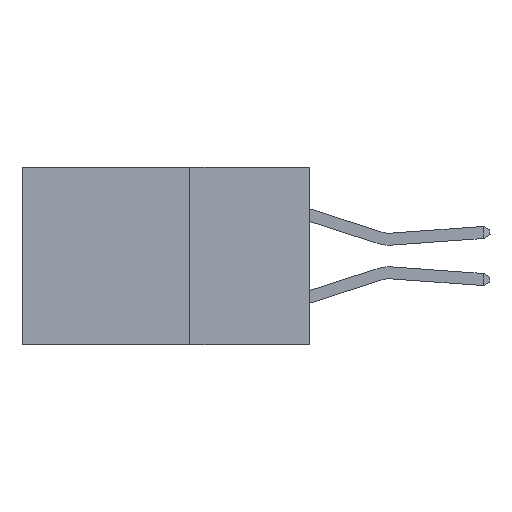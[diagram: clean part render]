
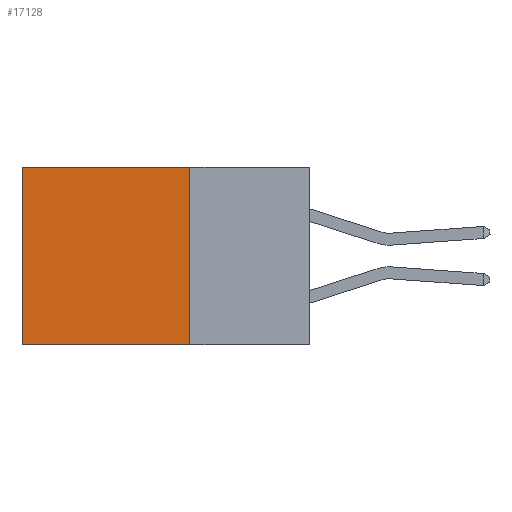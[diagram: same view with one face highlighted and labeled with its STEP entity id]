
A CAD part, left-side view. The second image highlights one B-rep face of the part: STEP entity #17128.
In plain terms, the highlighted planar face has unit normal (-1, 0, 0).
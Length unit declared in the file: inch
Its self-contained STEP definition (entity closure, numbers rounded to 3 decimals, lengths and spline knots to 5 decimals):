
#184 = LINE ( 'NONE', #22517, #8501 ) ;
#696 = CARTESIAN_POINT ( 'NONE',  ( 0.298, 0.6, 0. ) ) ;
#2286 = EDGE_CURVE ( 'NONE', #18534, #9116, #24153, .T. ) ;
#2993 = DIRECTION ( 'NONE',  ( 0., 0., -1. ) ) ;
#3890 = DIRECTION ( 'NONE',  ( 0., 0., -1. ) ) ;
#3920 = VECTOR ( 'NONE', #28299, 39.37008 ) ;
#4253 = EDGE_LOOP ( 'NONE', ( #7349, #31190, #12575, #24698 ) ) ;
#7349 = ORIENTED_EDGE ( 'NONE', *, *, #2286, .T. ) ;
#8501 = VECTOR ( 'NONE', #25023, 39.37008 ) ;
#9116 = VERTEX_POINT ( 'NONE', #18251 ) ;
#9934 = EDGE_CURVE ( 'NONE', #31045, #18534, #184, .T. ) ;
#10571 = CARTESIAN_POINT ( 'NONE',  ( 0.298, 0.25, 0. ) ) ;
#11083 = AXIS2_PLACEMENT_3D ( 'NONE', #10571, #18210, #2993 ) ;
#12575 = ORIENTED_EDGE ( 'NONE', *, *, #26874, .F. ) ;
#14338 = FACE_OUTER_BOUND ( 'NONE', #4253, .T. ) ;
#14443 = CARTESIAN_POINT ( 'NONE',  ( 0.298, 0.25, -0.37 ) ) ;
#15634 = PLANE ( 'NONE',  #11083 ) ;
#17128 = ADVANCED_FACE ( 'NONE', ( #14338 ), #15634, .F. ) ;
#17450 = VECTOR ( 'NONE', #3890, 39.37008 ) ;
#18210 = DIRECTION ( 'NONE',  ( 1., 0., 0. ) ) ;
#18235 = CARTESIAN_POINT ( 'NONE',  ( 0.298, 0.6, 0. ) ) ;
#18249 = LINE ( 'NONE', #19089, #17450 ) ;
#18251 = CARTESIAN_POINT ( 'NONE',  ( 0.298, 0.6, -0.37 ) ) ;
#18534 = VERTEX_POINT ( 'NONE', #18235 ) ;
#19089 = CARTESIAN_POINT ( 'NONE',  ( 0.298, 0.25, 0. ) ) ;
#21722 = VECTOR ( 'NONE', #27065, 39.37008 ) ;
#22517 = CARTESIAN_POINT ( 'NONE',  ( 0.298, 0.25, 0. ) ) ;
#22523 = LINE ( 'NONE', #14443, #21722 ) ;
#24153 = LINE ( 'NONE', #696, #3920 ) ;
#24698 = ORIENTED_EDGE ( 'NONE', *, *, #9934, .T. ) ;
#25023 = DIRECTION ( 'NONE',  ( 0., 1., 0. ) ) ;
#26874 = EDGE_CURVE ( 'NONE', #31045, #28324, #18249, .T. ) ;
#27065 = DIRECTION ( 'NONE',  ( 0., 1., 0. ) ) ;
#28202 = EDGE_CURVE ( 'NONE', #28324, #9116, #22523, .T. ) ;
#28299 = DIRECTION ( 'NONE',  ( 0., 0., -1. ) ) ;
#28324 = VERTEX_POINT ( 'NONE', #30113 ) ;
#29826 = CARTESIAN_POINT ( 'NONE',  ( 0.298, 0.25, 0. ) ) ;
#30113 = CARTESIAN_POINT ( 'NONE',  ( 0.298, 0.25, -0.37 ) ) ;
#31045 = VERTEX_POINT ( 'NONE', #29826 ) ;
#31190 = ORIENTED_EDGE ( 'NONE', *, *, #28202, .F. ) ;
